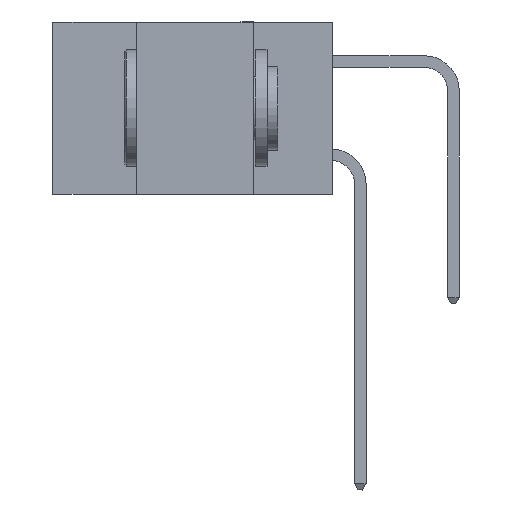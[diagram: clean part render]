
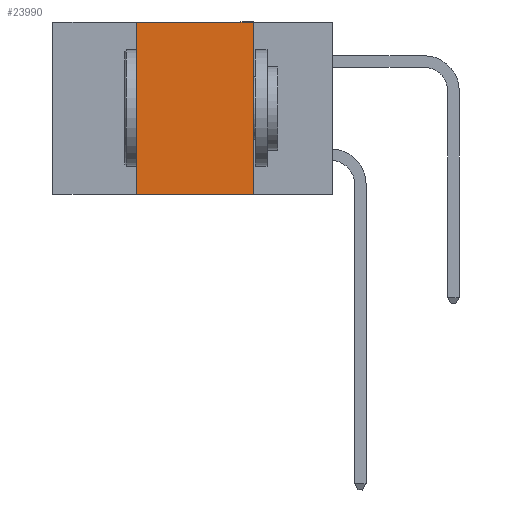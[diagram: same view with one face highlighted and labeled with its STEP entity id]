
A CAD part, left-side view. The second image highlights one B-rep face of the part: STEP entity #23990.
In plain terms, the highlighted planar face has unit normal (-1, 0, 0).
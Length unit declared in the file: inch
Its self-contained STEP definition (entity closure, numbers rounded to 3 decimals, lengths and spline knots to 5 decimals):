
#203 = CARTESIAN_POINT ( 'NONE',  ( 0., 0.6, -0.37 ) ) ;
#636 = ORIENTED_EDGE ( 'NONE', *, *, #9965, .F. ) ;
#1198 = EDGE_LOOP ( 'NONE', ( #21077, #636, #21093, #17702 ) ) ;
#1729 = CARTESIAN_POINT ( 'NONE',  ( 0., 0.17, -0.37 ) ) ;
#3741 = DIRECTION ( 'NONE',  ( 0., -1., 0. ) ) ;
#3799 = VECTOR ( 'NONE', #11907, 39.37008 ) ;
#5572 = DIRECTION ( 'NONE',  ( 0., 0., -1. ) ) ;
#6104 = CARTESIAN_POINT ( 'NONE',  ( 0., 0.17, 0. ) ) ;
#6205 = CARTESIAN_POINT ( 'NONE',  ( 0., 0.42, 0. ) ) ;
#7286 = LINE ( 'NONE', #6205, #3799 ) ;
#7378 = PLANE ( 'NONE',  #21235 ) ;
#7730 = DIRECTION ( 'NONE',  ( 0., 0., -1. ) ) ;
#8209 = EDGE_CURVE ( 'NONE', #16179, #10750, #16804, .T. ) ;
#8919 = DIRECTION ( 'NONE',  ( 1., 0., 0. ) ) ;
#9020 = DIRECTION ( 'NONE',  ( 0., -1., 0. ) ) ;
#9757 = VECTOR ( 'NONE', #3741, 39.37008 ) ;
#9965 = EDGE_CURVE ( 'NONE', #23707, #16179, #11718, .T. ) ;
#10280 = VECTOR ( 'NONE', #9020, 39.37008 ) ;
#10394 = CARTESIAN_POINT ( 'NONE',  ( 0., 0.42, 0. ) ) ;
#10750 = VERTEX_POINT ( 'NONE', #1729 ) ;
#11718 = LINE ( 'NONE', #20035, #10280 ) ;
#11907 = DIRECTION ( 'NONE',  ( 0., 0., 1. ) ) ;
#14240 = EDGE_CURVE ( 'NONE', #20510, #10750, #23153, .T. ) ;
#15009 = CARTESIAN_POINT ( 'NONE',  ( 0., 0.17, 0. ) ) ;
#16179 = VERTEX_POINT ( 'NONE', #15009 ) ;
#16804 = LINE ( 'NONE', #6104, #21141 ) ;
#17702 = ORIENTED_EDGE ( 'NONE', *, *, #14240, .T. ) ;
#17808 = CARTESIAN_POINT ( 'NONE',  ( 0., 0.42, -0.37 ) ) ;
#19434 = CARTESIAN_POINT ( 'NONE',  ( 0., 0.6, 0. ) ) ;
#20035 = CARTESIAN_POINT ( 'NONE',  ( 0., 0.6, 0. ) ) ;
#20510 = VERTEX_POINT ( 'NONE', #17808 ) ;
#21077 = ORIENTED_EDGE ( 'NONE', *, *, #8209, .F. ) ;
#21093 = ORIENTED_EDGE ( 'NONE', *, *, #23938, .F. ) ;
#21141 = VECTOR ( 'NONE', #7730, 39.37008 ) ;
#21235 = AXIS2_PLACEMENT_3D ( 'NONE', #19434, #8919, #5572 ) ;
#23025 = FACE_OUTER_BOUND ( 'NONE', #1198, .T. ) ;
#23153 = LINE ( 'NONE', #203, #9757 ) ;
#23707 = VERTEX_POINT ( 'NONE', #10394 ) ;
#23938 = EDGE_CURVE ( 'NONE', #20510, #23707, #7286, .T. ) ;
#23990 = ADVANCED_FACE ( 'NONE', ( #23025 ), #7378, .F. ) ;
